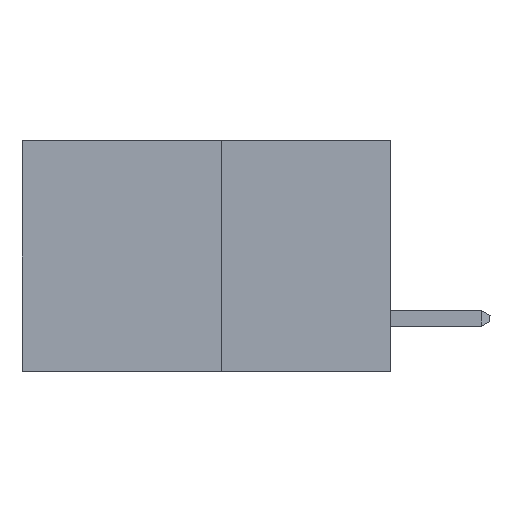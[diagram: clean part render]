
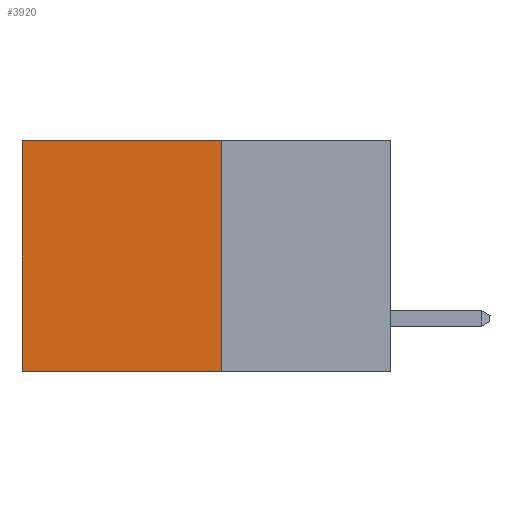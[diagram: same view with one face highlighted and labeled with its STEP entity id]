
A CAD part, left-side view. The second image highlights one B-rep face of the part: STEP entity #3920.
In plain terms, the highlighted planar face has unit normal (-1, 0, 0).
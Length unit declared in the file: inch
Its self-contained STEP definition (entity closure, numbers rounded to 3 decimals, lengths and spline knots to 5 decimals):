
#50 = FACE_OUTER_BOUND ( 'NONE', #6188, .T. ) ;
#235 = VERTEX_POINT ( 'NONE', #6705 ) ;
#409 = DIRECTION ( 'NONE',  ( 1., 0., 0. ) ) ;
#495 = EDGE_CURVE ( 'NONE', #7959, #6176, #6272, .T. ) ;
#563 = PLANE ( 'NONE',  #5495 ) ;
#622 = VECTOR ( 'NONE', #1805, 39.37008 ) ;
#627 = CARTESIAN_POINT ( 'NONE',  ( 0.277, 0.27, 0. ) ) ;
#664 = DIRECTION ( 'NONE',  ( 0., 1., 0. ) ) ;
#794 = EDGE_CURVE ( 'NONE', #235, #3113, #6667, .T. ) ;
#1805 = DIRECTION ( 'NONE',  ( 0., 0., -1. ) ) ;
#2019 = DIRECTION ( 'NONE',  ( 0., 0., -1. ) ) ;
#2231 = ORIENTED_EDGE ( 'NONE', *, *, #5150, .T. ) ;
#2540 = EDGE_CURVE ( 'NONE', #7959, #235, #8046, .T. ) ;
#3113 = VERTEX_POINT ( 'NONE', #4589 ) ;
#3173 = CARTESIAN_POINT ( 'NONE',  ( 0.277, 0.59, 0. ) ) ;
#3690 = CARTESIAN_POINT ( 'NONE',  ( 0.277, 0.27, -0.37 ) ) ;
#3920 = ADVANCED_FACE ( 'NONE', ( #50 ), #563, .F. ) ;
#4312 = ORIENTED_EDGE ( 'NONE', *, *, #495, .T. ) ;
#4319 = ORIENTED_EDGE ( 'NONE', *, *, #794, .F. ) ;
#4573 = ORIENTED_EDGE ( 'NONE', *, *, #2540, .F. ) ;
#4589 = CARTESIAN_POINT ( 'NONE',  ( 0.277, 0.59, -0.37 ) ) ;
#5019 = VECTOR ( 'NONE', #8578, 39.37008 ) ;
#5093 = CARTESIAN_POINT ( 'NONE',  ( 0.277, 0.59, -0.37 ) ) ;
#5110 = DIRECTION ( 'NONE',  ( 0., 0., -1. ) ) ;
#5150 = EDGE_CURVE ( 'NONE', #6176, #3113, #7658, .T. ) ;
#5495 = AXIS2_PLACEMENT_3D ( 'NONE', #8952, #409, #2019 ) ;
#5575 = VECTOR ( 'NONE', #5110, 39.37008 ) ;
#6176 = VERTEX_POINT ( 'NONE', #3173 ) ;
#6188 = EDGE_LOOP ( 'NONE', ( #2231, #4319, #4573, #4312 ) ) ;
#6272 = LINE ( 'NONE', #627, #7701 ) ;
#6667 = LINE ( 'NONE', #8638, #5019 ) ;
#6705 = CARTESIAN_POINT ( 'NONE',  ( 0.277, 0.27, -0.37 ) ) ;
#7071 = CARTESIAN_POINT ( 'NONE',  ( 0.277, 0.27, 0. ) ) ;
#7658 = LINE ( 'NONE', #5093, #5575 ) ;
#7701 = VECTOR ( 'NONE', #664, 39.37008 ) ;
#7959 = VERTEX_POINT ( 'NONE', #7071 ) ;
#8046 = LINE ( 'NONE', #3690, #622 ) ;
#8578 = DIRECTION ( 'NONE',  ( 0., 1., 0. ) ) ;
#8638 = CARTESIAN_POINT ( 'NONE',  ( 0.277, 0.27, -0.37 ) ) ;
#8952 = CARTESIAN_POINT ( 'NONE',  ( 0.277, 0.27, -0.37 ) ) ;
